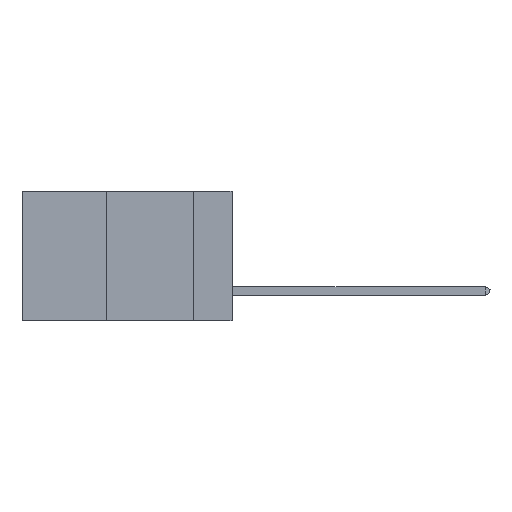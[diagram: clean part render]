
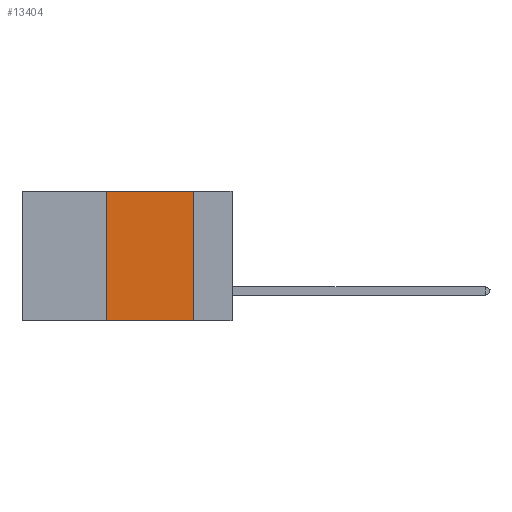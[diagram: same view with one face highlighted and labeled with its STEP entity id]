
A CAD part, left-side view. The second image highlights one B-rep face of the part: STEP entity #13404.
In plain terms, the highlighted planar face has unit normal (-1, 0, 0).
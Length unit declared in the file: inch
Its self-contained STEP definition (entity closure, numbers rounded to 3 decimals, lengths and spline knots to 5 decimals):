
#1338 = DIRECTION ( 'NONE',  ( 1., 0., 0. ) ) ;
#1821 = VERTEX_POINT ( 'NONE', #17222 ) ;
#2514 = CARTESIAN_POINT ( 'NONE',  ( 0., 0.36, 0. ) ) ;
#2769 = LINE ( 'NONE', #6571, #7076 ) ;
#3141 = DIRECTION ( 'NONE',  ( 0., 0., -1. ) ) ;
#4693 = LINE ( 'NONE', #19109, #15755 ) ;
#5039 = VERTEX_POINT ( 'NONE', #21955 ) ;
#5053 = AXIS2_PLACEMENT_3D ( 'NONE', #16162, #1338, #3141 ) ;
#5506 = VERTEX_POINT ( 'NONE', #2514 ) ;
#5943 = EDGE_CURVE ( 'NONE', #5039, #5506, #10476, .T. ) ;
#6571 = CARTESIAN_POINT ( 'NONE',  ( 0., 0.6, 0. ) ) ;
#7076 = VECTOR ( 'NONE', #15572, 39.37008 ) ;
#7251 = EDGE_CURVE ( 'NONE', #5039, #1821, #4693, .T. ) ;
#8352 = DIRECTION ( 'NONE',  ( 0., -1., 0. ) ) ;
#9328 = EDGE_LOOP ( 'NONE', ( #22376, #19445, #18745, #18522 ) ) ;
#9584 = VERTEX_POINT ( 'NONE', #15478 ) ;
#10476 = LINE ( 'NONE', #19561, #15794 ) ;
#11123 = EDGE_CURVE ( 'NONE', #5506, #9584, #2769, .T. ) ;
#12884 = EDGE_CURVE ( 'NONE', #9584, #1821, #20269, .T. ) ;
#13404 = ADVANCED_FACE ( 'NONE', ( #15381 ), #22781, .F. ) ;
#14002 = VECTOR ( 'NONE', #17618, 39.37008 ) ;
#15381 = FACE_OUTER_BOUND ( 'NONE', #9328, .T. ) ;
#15478 = CARTESIAN_POINT ( 'NONE',  ( 0., 0.11, 0. ) ) ;
#15572 = DIRECTION ( 'NONE',  ( 0., -1., 0. ) ) ;
#15755 = VECTOR ( 'NONE', #8352, 39.37008 ) ;
#15794 = VECTOR ( 'NONE', #21547, 39.37008 ) ;
#16162 = CARTESIAN_POINT ( 'NONE',  ( 0., 0.6, 0. ) ) ;
#16415 = CARTESIAN_POINT ( 'NONE',  ( 0., 0.11, 0. ) ) ;
#17222 = CARTESIAN_POINT ( 'NONE',  ( 0., 0.11, -0.37 ) ) ;
#17618 = DIRECTION ( 'NONE',  ( 0., 0., -1. ) ) ;
#18522 = ORIENTED_EDGE ( 'NONE', *, *, #7251, .T. ) ;
#18745 = ORIENTED_EDGE ( 'NONE', *, *, #5943, .F. ) ;
#19109 = CARTESIAN_POINT ( 'NONE',  ( 0., 0.6, -0.37 ) ) ;
#19445 = ORIENTED_EDGE ( 'NONE', *, *, #11123, .F. ) ;
#19561 = CARTESIAN_POINT ( 'NONE',  ( 0., 0.36, 0. ) ) ;
#20269 = LINE ( 'NONE', #16415, #14002 ) ;
#21547 = DIRECTION ( 'NONE',  ( 0., 0., 1. ) ) ;
#21955 = CARTESIAN_POINT ( 'NONE',  ( 0., 0.36, -0.37 ) ) ;
#22376 = ORIENTED_EDGE ( 'NONE', *, *, #12884, .F. ) ;
#22781 = PLANE ( 'NONE',  #5053 ) ;
